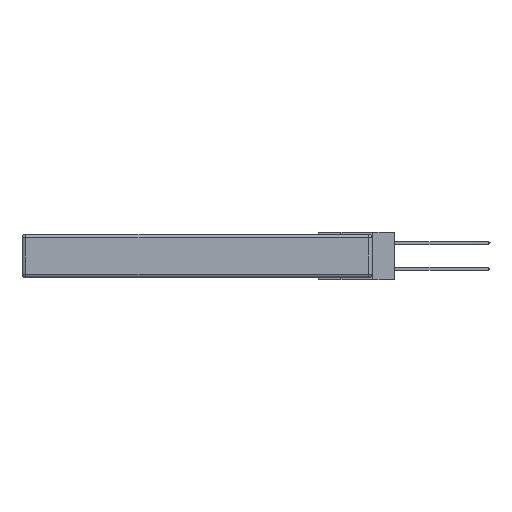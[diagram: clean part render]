
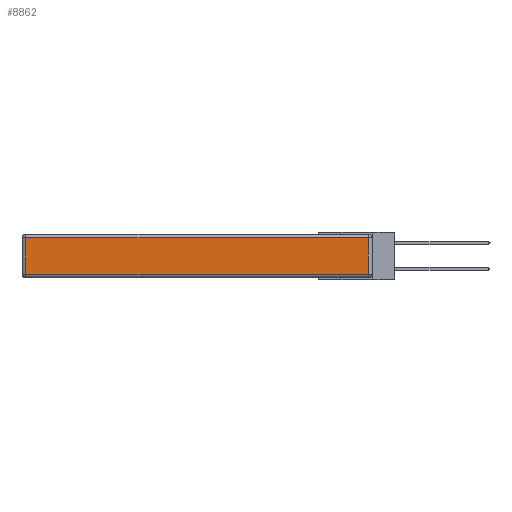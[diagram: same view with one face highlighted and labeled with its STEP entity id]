
A CAD part, left-side view. The second image highlights one B-rep face of the part: STEP entity #8862.
In plain terms, the highlighted planar face has unit normal (-1, 0, 0).
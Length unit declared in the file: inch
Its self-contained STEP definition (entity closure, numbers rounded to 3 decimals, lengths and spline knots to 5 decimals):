
#424 = EDGE_CURVE ( 'NONE', #5405, #3740, #7982, .T. ) ;
#1161 = EDGE_CURVE ( 'NONE', #3740, #2394, #8755, .T. ) ;
#1371 = AXIS2_PLACEMENT_3D ( 'NONE', #13279, #15954, #14564 ) ;
#1958 = CARTESIAN_POINT ( 'NONE',  ( 0., 0., -0.313 ) ) ;
#2148 = ORIENTED_EDGE ( 'NONE', *, *, #1161, .T. ) ;
#2394 = VERTEX_POINT ( 'NONE', #3700 ) ;
#2460 = CARTESIAN_POINT ( 'NONE',  ( 0., 0.03, -0.313 ) ) ;
#3049 = DIRECTION ( 'NONE',  ( 0., 0., 1. ) ) ;
#3443 = LINE ( 'NONE', #1958, #16203 ) ;
#3700 = CARTESIAN_POINT ( 'NONE',  ( 0., 2.72, -0.03 ) ) ;
#3740 = VERTEX_POINT ( 'NONE', #13200 ) ;
#4170 = PLANE ( 'NONE',  #1371 ) ;
#4334 = DIRECTION ( 'NONE',  ( 0., 1., 0. ) ) ;
#5405 = VERTEX_POINT ( 'NONE', #2460 ) ;
#5411 = FACE_OUTER_BOUND ( 'NONE', #11155, .T. ) ;
#6341 = EDGE_CURVE ( 'NONE', #11825, #5405, #3443, .T. ) ;
#7982 = LINE ( 'NONE', #12138, #12409 ) ;
#8755 = LINE ( 'NONE', #12134, #16032 ) ;
#8862 = ADVANCED_FACE ( 'NONE', ( #5411 ), #4170, .T. ) ;
#10447 = DIRECTION ( 'NONE',  ( 0., -1., 0. ) ) ;
#10855 = ORIENTED_EDGE ( 'NONE', *, *, #6341, .T. ) ;
#10997 = CARTESIAN_POINT ( 'NONE',  ( 0., 2.72, -0.313 ) ) ;
#11155 = EDGE_LOOP ( 'NONE', ( #10855, #16385, #2148, #15972 ) ) ;
#11825 = VERTEX_POINT ( 'NONE', #10997 ) ;
#12134 = CARTESIAN_POINT ( 'NONE',  ( 0., 2.75, -0.03 ) ) ;
#12138 = CARTESIAN_POINT ( 'NONE',  ( 0., 0.03, -0.343 ) ) ;
#12139 = VECTOR ( 'NONE', #13571, 39.37008 ) ;
#12409 = VECTOR ( 'NONE', #3049, 39.37008 ) ;
#12952 = LINE ( 'NONE', #16255, #12139 ) ;
#13200 = CARTESIAN_POINT ( 'NONE',  ( 0., 0.03, -0.03 ) ) ;
#13279 = CARTESIAN_POINT ( 'NONE',  ( 0., 0., -0.343 ) ) ;
#13571 = DIRECTION ( 'NONE',  ( 0., 0., -1. ) ) ;
#13642 = EDGE_CURVE ( 'NONE', #2394, #11825, #12952, .T. ) ;
#14564 = DIRECTION ( 'NONE',  ( 0., 0., 1. ) ) ;
#15954 = DIRECTION ( 'NONE',  ( -1., 0., 0. ) ) ;
#15972 = ORIENTED_EDGE ( 'NONE', *, *, #13642, .T. ) ;
#16032 = VECTOR ( 'NONE', #4334, 39.37008 ) ;
#16203 = VECTOR ( 'NONE', #10447, 39.37008 ) ;
#16255 = CARTESIAN_POINT ( 'NONE',  ( 0., 2.72, -0.343 ) ) ;
#16385 = ORIENTED_EDGE ( 'NONE', *, *, #424, .T. ) ;
